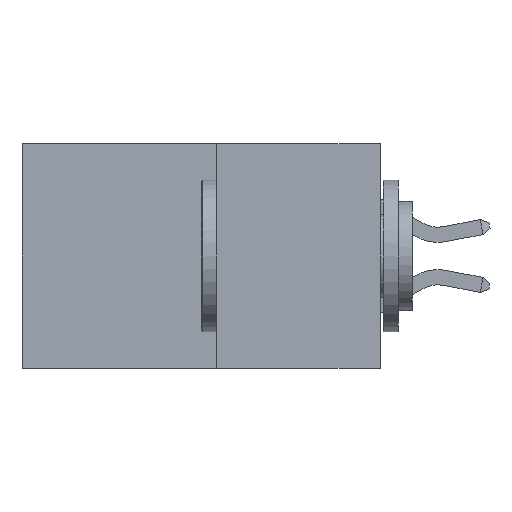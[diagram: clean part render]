
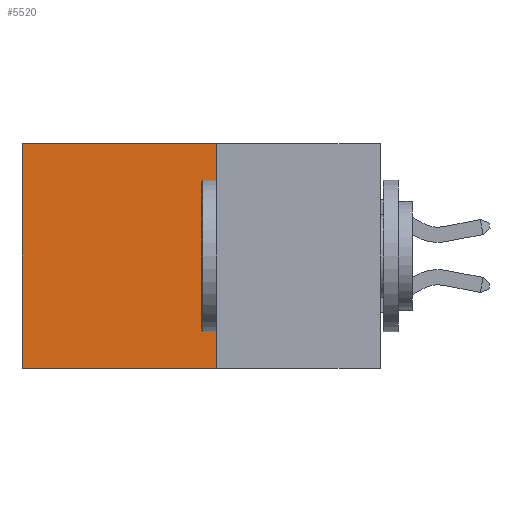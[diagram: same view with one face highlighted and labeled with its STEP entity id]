
A CAD part, left-side view. The second image highlights one B-rep face of the part: STEP entity #5520.
In plain terms, the highlighted planar face has unit normal (-1, 0, 0).
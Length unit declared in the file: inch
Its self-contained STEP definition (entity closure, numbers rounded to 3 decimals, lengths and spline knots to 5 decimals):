
#64 = ORIENTED_EDGE ( 'NONE', *, *, #1263, .T. ) ;
#1033 = LINE ( 'NONE', #1337, #6236 ) ;
#1040 = DIRECTION ( 'NONE',  ( 1., 0., 0. ) ) ;
#1044 = EDGE_CURVE ( 'NONE', #2567, #1079, #8449, .T. ) ;
#1079 = VERTEX_POINT ( 'NONE', #1252 ) ;
#1252 = CARTESIAN_POINT ( 'NONE',  ( 0.277, 0.59, -0.37 ) ) ;
#1263 = EDGE_CURVE ( 'NONE', #7015, #2457, #1721, .T. ) ;
#1337 = CARTESIAN_POINT ( 'NONE',  ( 0.277, 0.27, -0.37 ) ) ;
#1721 = LINE ( 'NONE', #6408, #8540 ) ;
#1895 = CARTESIAN_POINT ( 'NONE',  ( 0.277, 0.27, 0. ) ) ;
#1912 = CARTESIAN_POINT ( 'NONE',  ( 0.277, 0.27, -0.37 ) ) ;
#2457 = VERTEX_POINT ( 'NONE', #3824 ) ;
#2567 = VERTEX_POINT ( 'NONE', #1912 ) ;
#3455 = EDGE_CURVE ( 'NONE', #7015, #2567, #1033, .T. ) ;
#3608 = DIRECTION ( 'NONE',  ( 0., 0., -1. ) ) ;
#3733 = DIRECTION ( 'NONE',  ( 0., 1., 0. ) ) ;
#3824 = CARTESIAN_POINT ( 'NONE',  ( 0.277, 0.59, 0. ) ) ;
#4017 = VECTOR ( 'NONE', #3608, 39.37008 ) ;
#4026 = ORIENTED_EDGE ( 'NONE', *, *, #6555, .T. ) ;
#4214 = FACE_OUTER_BOUND ( 'NONE', #5225, .T. ) ;
#4235 = LINE ( 'NONE', #7532, #4017 ) ;
#4243 = DIRECTION ( 'NONE',  ( 0., 0., -1. ) ) ;
#4603 = DIRECTION ( 'NONE',  ( 0., 1., 0. ) ) ;
#5109 = ORIENTED_EDGE ( 'NONE', *, *, #1044, .F. ) ;
#5225 = EDGE_LOOP ( 'NONE', ( #4026, #5109, #8444, #64 ) ) ;
#5520 = ADVANCED_FACE ( 'NONE', ( #4214 ), #6426, .F. ) ;
#5776 = CARTESIAN_POINT ( 'NONE',  ( 0.277, 0.27, -0.37 ) ) ;
#5804 = DIRECTION ( 'NONE',  ( 0., 0., -1. ) ) ;
#6236 = VECTOR ( 'NONE', #4243, 39.37008 ) ;
#6408 = CARTESIAN_POINT ( 'NONE',  ( 0.277, 0.27, 0. ) ) ;
#6426 = PLANE ( 'NONE',  #6678 ) ;
#6555 = EDGE_CURVE ( 'NONE', #2457, #1079, #4235, .T. ) ;
#6678 = AXIS2_PLACEMENT_3D ( 'NONE', #5776, #1040, #5804 ) ;
#6715 = CARTESIAN_POINT ( 'NONE',  ( 0.277, 0.27, -0.37 ) ) ;
#7015 = VERTEX_POINT ( 'NONE', #1895 ) ;
#7532 = CARTESIAN_POINT ( 'NONE',  ( 0.277, 0.59, -0.37 ) ) ;
#8245 = VECTOR ( 'NONE', #4603, 39.37008 ) ;
#8444 = ORIENTED_EDGE ( 'NONE', *, *, #3455, .F. ) ;
#8449 = LINE ( 'NONE', #6715, #8245 ) ;
#8540 = VECTOR ( 'NONE', #3733, 39.37008 ) ;
